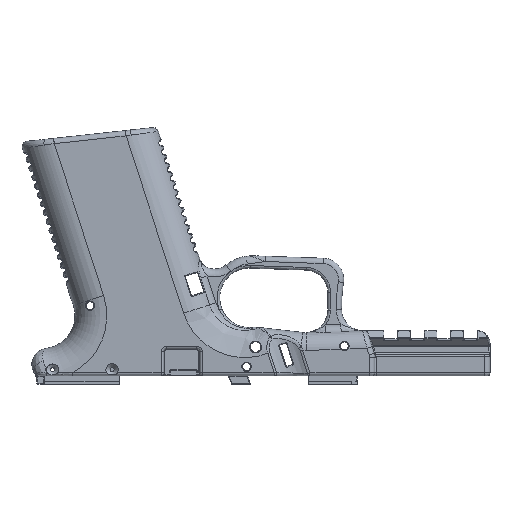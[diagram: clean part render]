
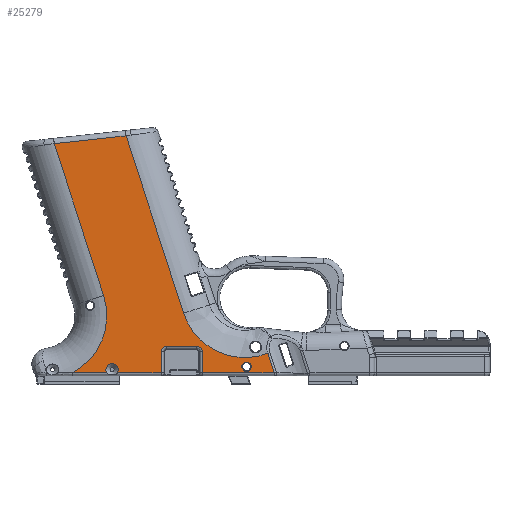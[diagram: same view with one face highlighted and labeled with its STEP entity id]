
A CAD part, front view. The second image highlights one B-rep face of the part: STEP entity #25279.
In plain terms, the highlighted planar face has unit normal (0, -1, 0).
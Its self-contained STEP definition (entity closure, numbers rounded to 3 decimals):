
#1282=FACE_BOUND('',#5088,.T.);
#1299=B_SPLINE_CURVE_WITH_KNOTS('',3,(#37240,#37241,#37242,#37243,#37244,
#37245,#37246),.UNSPECIFIED.,.F.,.F.,(4,1,1,1,4),(0.,0.617,
1.85,3.084,3.929),.UNSPECIFIED.);
#3404=FACE_OUTER_BOUND('',#5087,.T.);
#5087=EDGE_LOOP('',(#20844,#20845,#20846,#20847,#20848,#20849,#20850,#20851,
#20852,#20853,#20854,#20855,#20856,#20857,#20858,#20859));
#5088=EDGE_LOOP('',(#20860));
#6177=CIRCLE('',#26982,2.312);
#6179=CIRCLE('',#26984,2.312);
#6582=CIRCLE('',#27791,1.749);
#6583=CIRCLE('',#27793,2.);
#6584=CIRCLE('',#27794,2.);
#6585=CIRCLE('',#27795,24.459);
#7594=LINE('',#43411,#9031);
#7667=LINE('',#48017,#9104);
#7715=LINE('',#48520,#9152);
#7716=LINE('',#48524,#9153);
#8108=LINE('',#54258,#9545);
#8109=LINE('',#54262,#9546);
#8110=LINE('',#54266,#9547);
#8111=LINE('',#54268,#9548);
#8112=LINE('',#54269,#9549);
#8113=LINE('',#54270,#9550);
#9031=VECTOR('',#30653,10.);
#9104=VECTOR('',#31260,10.);
#9152=VECTOR('',#31462,10.);
#9153=VECTOR('',#31467,10.);
#9545=VECTOR('',#33469,10.);
#9546=VECTOR('',#33472,10.);
#9547=VECTOR('',#33475,10.);
#9548=VECTOR('',#33476,10.);
#9549=VECTOR('',#33477,10.);
#9550=VECTOR('',#33478,10.);
#10256=VERTEX_POINT('',#37237);
#10257=VERTEX_POINT('',#37239);
#10703=VERTEX_POINT('',#43409);
#10930=VERTEX_POINT('',#48014);
#10931=VERTEX_POINT('',#48016);
#10997=VERTEX_POINT('',#48492);
#10998=VERTEX_POINT('',#48493);
#10999=VERTEX_POINT('',#48512);
#11001=VERTEX_POINT('',#48519);
#11002=VERTEX_POINT('',#48522);
#11579=VERTEX_POINT('',#54253);
#11580=VERTEX_POINT('',#54257);
#11581=VERTEX_POINT('',#54259);
#11582=VERTEX_POINT('',#54261);
#11583=VERTEX_POINT('',#54263);
#11584=VERTEX_POINT('',#54265);
#11585=VERTEX_POINT('',#54267);
#12566=EDGE_CURVE('',#10256,#10257,#1299,.T.);
#13264=EDGE_CURVE('',#10703,#10256,#7594,.T.);
#13657=EDGE_CURVE('',#10930,#10931,#7667,.T.);
#13759=EDGE_CURVE('',#10998,#10999,#6177,.T.);
#13762=EDGE_CURVE('',#10999,#10997,#6179,.T.);
#13763=EDGE_CURVE('',#10997,#11001,#7715,.T.);
#13766=EDGE_CURVE('',#11002,#10998,#7716,.T.);
#14782=EDGE_CURVE('',#11579,#11579,#6582,.T.);
#14784=EDGE_CURVE('',#11580,#11002,#8108,.T.);
#14785=EDGE_CURVE('',#11581,#11580,#6583,.T.);
#14786=EDGE_CURVE('',#11582,#11581,#8109,.T.);
#14787=EDGE_CURVE('',#11583,#11582,#6584,.T.);
#14788=EDGE_CURVE('',#11584,#11583,#8110,.T.);
#14789=EDGE_CURVE('',#11585,#11584,#8111,.T.);
#14790=EDGE_CURVE('',#10257,#11585,#8112,.T.);
#14791=EDGE_CURVE('',#10931,#10703,#8113,.T.);
#14792=EDGE_CURVE('',#11001,#10930,#6585,.T.);
#20844=ORIENTED_EDGE('',*,*,#13759,.F.);
#20845=ORIENTED_EDGE('',*,*,#13766,.F.);
#20846=ORIENTED_EDGE('',*,*,#14784,.F.);
#20847=ORIENTED_EDGE('',*,*,#14785,.F.);
#20848=ORIENTED_EDGE('',*,*,#14786,.F.);
#20849=ORIENTED_EDGE('',*,*,#14787,.F.);
#20850=ORIENTED_EDGE('',*,*,#14788,.F.);
#20851=ORIENTED_EDGE('',*,*,#14789,.F.);
#20852=ORIENTED_EDGE('',*,*,#14790,.F.);
#20853=ORIENTED_EDGE('',*,*,#12566,.F.);
#20854=ORIENTED_EDGE('',*,*,#13264,.F.);
#20855=ORIENTED_EDGE('',*,*,#14791,.F.);
#20856=ORIENTED_EDGE('',*,*,#13657,.F.);
#20857=ORIENTED_EDGE('',*,*,#14792,.F.);
#20858=ORIENTED_EDGE('',*,*,#13763,.F.);
#20859=ORIENTED_EDGE('',*,*,#13762,.F.);
#20860=ORIENTED_EDGE('',*,*,#14782,.F.);
#24203=PLANE('',#27792);
#25279=ADVANCED_FACE('',(#3404,#1282),#24203,.F.);
#26982=AXIS2_PLACEMENT_3D('',#48513,#31453,#31454);
#26984=AXIS2_PLACEMENT_3D('',#48517,#31458,#31459);
#27791=AXIS2_PLACEMENT_3D('',#54254,#33464,#33465);
#27792=AXIS2_PLACEMENT_3D('',#54256,#33467,#33468);
#27793=AXIS2_PLACEMENT_3D('',#54260,#33470,#33471);
#27794=AXIS2_PLACEMENT_3D('',#54264,#33473,#33474);
#27795=AXIS2_PLACEMENT_3D('',#54271,#33479,#33480);
#30653=DIRECTION('',(0.309,0.,-0.951));
#31260=DIRECTION('',(-0.309,0.,0.951));
#31453=DIRECTION('center_axis',(0.,-1.,0.));
#31454=DIRECTION('ref_axis',(-1.,0.,0.));
#31458=DIRECTION('center_axis',(0.,-1.,0.));
#31459=DIRECTION('ref_axis',(-1.,0.,0.));
#31462=DIRECTION('',(-1.,0.,0.));
#31467=DIRECTION('',(-1.,0.,0.));
#33464=DIRECTION('center_axis',(0.,-1.,0.));
#33465=DIRECTION('ref_axis',(1.,0.,0.));
#33467=DIRECTION('center_axis',(0.,1.,0.));
#33468=DIRECTION('ref_axis',(1.,0.,0.));
#33469=DIRECTION('',(0.,0.,-1.));
#33470=DIRECTION('center_axis',(0.,-1.,0.));
#33471=DIRECTION('ref_axis',(-0.707,0.,0.707));
#33472=DIRECTION('',(-1.,0.,0.));
#33473=DIRECTION('center_axis',(0.,-1.,0.));
#33474=DIRECTION('ref_axis',(0.707,0.,0.707));
#33475=DIRECTION('',(0.,0.,1.));
#33476=DIRECTION('',(-1.,0.,0.));
#33477=DIRECTION('',(0.309,0.,-0.951));
#33478=DIRECTION('',(0.994,0.,0.108));
#33479=DIRECTION('center_axis',(0.,-1.,0.));
#33480=DIRECTION('ref_axis',(0.864,0.,-0.504));
#37237=CARTESIAN_POINT('',(-22.508,-15.,-16.454));
#37239=CARTESIAN_POINT('',(9.188,-15.,-31.578));
#37240=CARTESIAN_POINT('Ctrl Pts',(-22.508,-15.,-16.454));
#37241=CARTESIAN_POINT('Ctrl Pts',(-21.873,-15.,-18.409));
#37242=CARTESIAN_POINT('Ctrl Pts',(-19.215,-15.,-24.033));
#37243=CARTESIAN_POINT('Ctrl Pts',(-11.431,-15.,-31.249));
#37244=CARTESIAN_POINT('Ctrl Pts',(-0.346,-15.,-33.947));
#37245=CARTESIAN_POINT('Ctrl Pts',(6.557,-15.,-32.587));
#37246=CARTESIAN_POINT('Ctrl Pts',(9.186,-15.,-31.576));
#43409=CARTESIAN_POINT('',(-44.24,-15.,50.429));
#43411=CARTESIAN_POINT('',(-45.977,-15.,55.774));
#48014=CARTESIAN_POINT('',(-52.712,-15.,-9.804));
#48016=CARTESIAN_POINT('',(-71.326,-15.,47.486));
#48017=CARTESIAN_POINT('',(-62.428,-15.,20.099));
#48492=CARTESIAN_POINT('',(-51.487,-15.,-39.));
#48493=CARTESIAN_POINT('',(-47.56,-15.,-39.));
#48512=CARTESIAN_POINT('',(-47.212,-15.,-37.78));
#48513=CARTESIAN_POINT('Origin',(-49.523,-15.,-37.78));
#48517=CARTESIAN_POINT('Origin',(-49.523,-15.,-37.78));
#48519=CARTESIAN_POINT('',(-64.57,-15.,-39.));
#48520=CARTESIAN_POINT('',(48.962,-15.,-39.));
#48522=CARTESIAN_POINT('',(-31.,-15.,-39.));
#48524=CARTESIAN_POINT('',(48.962,-15.,-39.));
#54253=CARTESIAN_POINT('',(-0.551,-15.,-36.614));
#54254=CARTESIAN_POINT('Origin',(1.197,-15.,-36.614));
#54256=CARTESIAN_POINT('Origin',(4.924,-15.,6.92));
#54257=CARTESIAN_POINT('',(-31.,-15.,-31.));
#54258=CARTESIAN_POINT('',(-31.,-15.,-16.54));
#54259=CARTESIAN_POINT('',(-29.,-15.,-29.));
#54260=CARTESIAN_POINT('Origin',(-29.,-15.,-31.));
#54261=CARTESIAN_POINT('',(-17.5,-15.,-29.));
#54262=CARTESIAN_POINT('',(-12.538,-15.,-29.));
#54263=CARTESIAN_POINT('',(-15.5,-15.,-31.));
#54264=CARTESIAN_POINT('Origin',(-17.5,-15.,-31.));
#54265=CARTESIAN_POINT('',(-15.5,-15.,-39.));
#54266=CARTESIAN_POINT('',(-15.5,-15.,-11.54));
#54267=CARTESIAN_POINT('',(11.599,-15.,-39.));
#54268=CARTESIAN_POINT('',(48.962,-15.,-39.));
#54269=CARTESIAN_POINT('',(8.701,-15.,-30.081));
#54270=CARTESIAN_POINT('',(-41.628,-15.,50.713));
#54271=CARTESIAN_POINT('Origin',(-75.974,-15.,-17.362));
